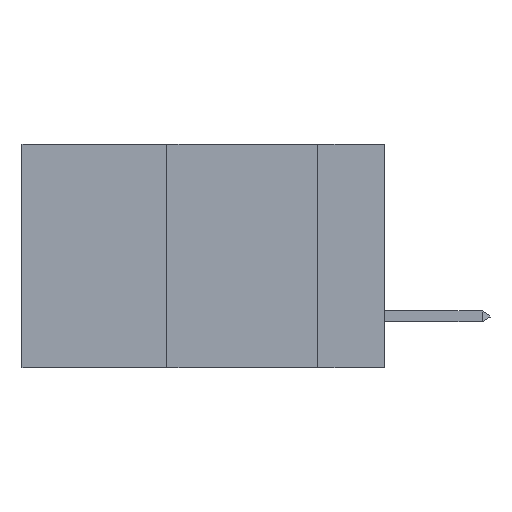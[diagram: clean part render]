
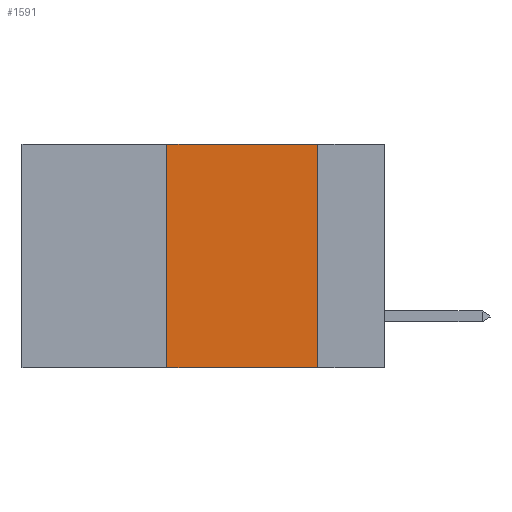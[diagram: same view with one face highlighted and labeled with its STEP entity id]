
A CAD part, left-side view. The second image highlights one B-rep face of the part: STEP entity #1591.
In plain terms, the highlighted planar face has unit normal (-1, 0, 0).
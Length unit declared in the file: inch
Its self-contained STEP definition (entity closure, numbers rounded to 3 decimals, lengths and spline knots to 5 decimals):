
#6 = DIRECTION ( 'NONE',  ( 0., 0., 1. ) ) ;
#74 = DIRECTION ( 'NONE',  ( 0., -1., 0. ) ) ;
#600 = DIRECTION ( 'NONE',  ( 0., 0., -1. ) ) ;
#751 = VERTEX_POINT ( 'NONE', #7768 ) ;
#816 = FACE_OUTER_BOUND ( 'NONE', #6831, .T. ) ;
#973 = VERTEX_POINT ( 'NONE', #8888 ) ;
#1059 = EDGE_CURVE ( 'NONE', #751, #4157, #8957, .T. ) ;
#1488 = PLANE ( 'NONE',  #3278 ) ;
#1492 = CARTESIAN_POINT ( 'NONE',  ( 0., 0.36, 0. ) ) ;
#1591 = ADVANCED_FACE ( 'NONE', ( #816 ), #1488, .F. ) ;
#1686 = ORIENTED_EDGE ( 'NONE', *, *, #5942, .F. ) ;
#2213 = CARTESIAN_POINT ( 'NONE',  ( 0., 0.6, 0. ) ) ;
#3017 = DIRECTION ( 'NONE',  ( 1., 0., 0. ) ) ;
#3114 = CARTESIAN_POINT ( 'NONE',  ( 0., 0.36, 0. ) ) ;
#3278 = AXIS2_PLACEMENT_3D ( 'NONE', #2213, #3017, #600 ) ;
#3400 = CARTESIAN_POINT ( 'NONE',  ( 0., 0.6, 0. ) ) ;
#4036 = DIRECTION ( 'NONE',  ( 0., -1., 0. ) ) ;
#4070 = VECTOR ( 'NONE', #74, 39.37008 ) ;
#4157 = VERTEX_POINT ( 'NONE', #1492 ) ;
#4313 = CARTESIAN_POINT ( 'NONE',  ( 0., 0.6, -0.37 ) ) ;
#4331 = CARTESIAN_POINT ( 'NONE',  ( 0., 0.11, 0. ) ) ;
#4944 = VECTOR ( 'NONE', #4036, 39.37008 ) ;
#5167 = VECTOR ( 'NONE', #6, 39.37008 ) ;
#5938 = EDGE_CURVE ( 'NONE', #6001, #973, #8674, .T. ) ;
#5942 = EDGE_CURVE ( 'NONE', #4157, #6001, #7688, .T. ) ;
#6001 = VERTEX_POINT ( 'NONE', #4331 ) ;
#6831 = EDGE_LOOP ( 'NONE', ( #7396, #1686, #7254, #9171 ) ) ;
#7254 = ORIENTED_EDGE ( 'NONE', *, *, #1059, .F. ) ;
#7396 = ORIENTED_EDGE ( 'NONE', *, *, #5938, .F. ) ;
#7688 = LINE ( 'NONE', #3400, #4070 ) ;
#7768 = CARTESIAN_POINT ( 'NONE',  ( 0., 0.36, -0.37 ) ) ;
#8661 = VECTOR ( 'NONE', #9012, 39.37008 ) ;
#8674 = LINE ( 'NONE', #8720, #8661 ) ;
#8720 = CARTESIAN_POINT ( 'NONE',  ( 0., 0.11, 0. ) ) ;
#8888 = CARTESIAN_POINT ( 'NONE',  ( 0., 0.11, -0.37 ) ) ;
#8957 = LINE ( 'NONE', #3114, #5167 ) ;
#8971 = EDGE_CURVE ( 'NONE', #751, #973, #9416, .T. ) ;
#9012 = DIRECTION ( 'NONE',  ( 0., 0., -1. ) ) ;
#9171 = ORIENTED_EDGE ( 'NONE', *, *, #8971, .T. ) ;
#9416 = LINE ( 'NONE', #4313, #4944 ) ;
